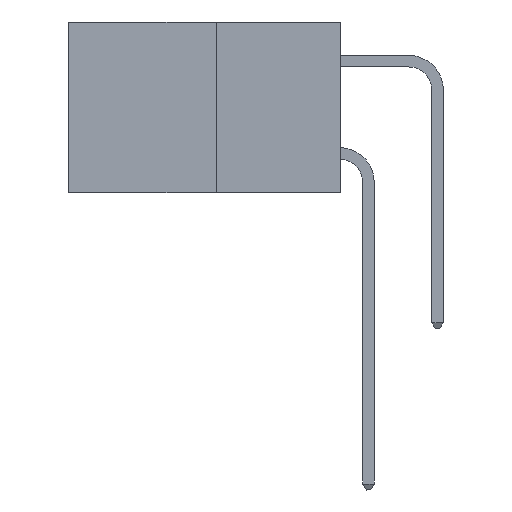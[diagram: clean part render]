
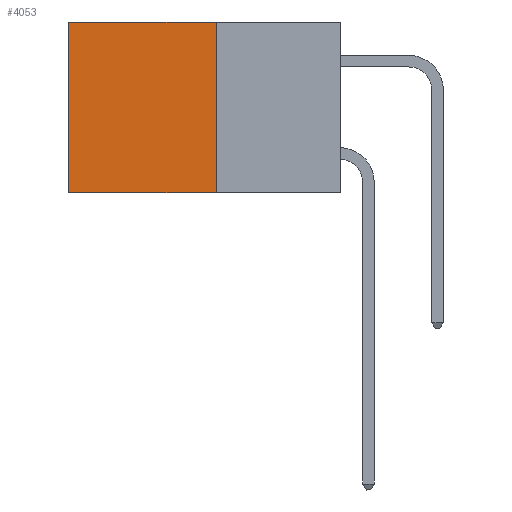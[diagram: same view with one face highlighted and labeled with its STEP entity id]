
A CAD part, left-side view. The second image highlights one B-rep face of the part: STEP entity #4053.
In plain terms, the highlighted planar face has unit normal (-1, 0, 0).
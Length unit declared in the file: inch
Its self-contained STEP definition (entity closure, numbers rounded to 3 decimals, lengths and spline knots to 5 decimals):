
#243 = EDGE_CURVE ( 'NONE', #8304, #2929, #3348, .T. ) ;
#590 = CARTESIAN_POINT ( 'NONE',  ( 0.277, 0.27, -0.37 ) ) ;
#743 = PLANE ( 'NONE',  #875 ) ;
#849 = VECTOR ( 'NONE', #1662, 39.37008 ) ;
#875 = AXIS2_PLACEMENT_3D ( 'NONE', #590, #992, #958 ) ;
#958 = DIRECTION ( 'NONE',  ( 0., 0., -1. ) ) ;
#992 = DIRECTION ( 'NONE',  ( 1., 0., 0. ) ) ;
#1176 = FACE_OUTER_BOUND ( 'NONE', #5696, .T. ) ;
#1336 = ORIENTED_EDGE ( 'NONE', *, *, #243, .T. ) ;
#1662 = DIRECTION ( 'NONE',  ( 0., 1., 0. ) ) ;
#2115 = VECTOR ( 'NONE', #5373, 39.37008 ) ;
#2274 = CARTESIAN_POINT ( 'NONE',  ( 0.277, 0.27, -0.37 ) ) ;
#2929 = VERTEX_POINT ( 'NONE', #8417 ) ;
#3348 = LINE ( 'NONE', #4088, #849 ) ;
#3537 = DIRECTION ( 'NONE',  ( 0., 0., -1. ) ) ;
#3540 = ORIENTED_EDGE ( 'NONE', *, *, #5922, .F. ) ;
#4053 = ADVANCED_FACE ( 'NONE', ( #1176 ), #743, .F. ) ;
#4088 = CARTESIAN_POINT ( 'NONE',  ( 0.277, 0.27, 0. ) ) ;
#4159 = VERTEX_POINT ( 'NONE', #2274 ) ;
#4611 = VECTOR ( 'NONE', #11381, 39.37008 ) ;
#5120 = CARTESIAN_POINT ( 'NONE',  ( 0.277, 0.27, -0.37 ) ) ;
#5373 = DIRECTION ( 'NONE',  ( 0., 0., -1. ) ) ;
#5696 = EDGE_LOOP ( 'NONE', ( #9983, #5738, #3540, #1336 ) ) ;
#5738 = ORIENTED_EDGE ( 'NONE', *, *, #9294, .F. ) ;
#5922 = EDGE_CURVE ( 'NONE', #8304, #4159, #6699, .T. ) ;
#6431 = CARTESIAN_POINT ( 'NONE',  ( 0.277, 0.27, 0. ) ) ;
#6699 = LINE ( 'NONE', #7268, #8850 ) ;
#7268 = CARTESIAN_POINT ( 'NONE',  ( 0.277, 0.27, -0.37 ) ) ;
#7452 = VERTEX_POINT ( 'NONE', #8063 ) ;
#7476 = EDGE_CURVE ( 'NONE', #2929, #7452, #9492, .T. ) ;
#8063 = CARTESIAN_POINT ( 'NONE',  ( 0.277, 0.59, -0.37 ) ) ;
#8304 = VERTEX_POINT ( 'NONE', #6431 ) ;
#8417 = CARTESIAN_POINT ( 'NONE',  ( 0.277, 0.59, 0. ) ) ;
#8850 = VECTOR ( 'NONE', #3537, 39.37008 ) ;
#9294 = EDGE_CURVE ( 'NONE', #4159, #7452, #11214, .T. ) ;
#9492 = LINE ( 'NONE', #9892, #2115 ) ;
#9892 = CARTESIAN_POINT ( 'NONE',  ( 0.277, 0.59, -0.37 ) ) ;
#9983 = ORIENTED_EDGE ( 'NONE', *, *, #7476, .T. ) ;
#11214 = LINE ( 'NONE', #5120, #4611 ) ;
#11381 = DIRECTION ( 'NONE',  ( 0., 1., 0. ) ) ;
